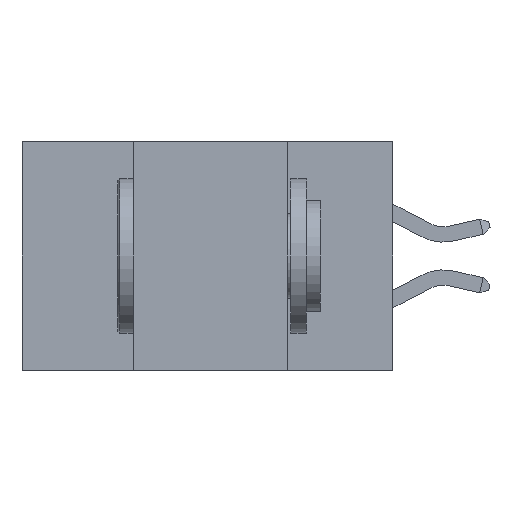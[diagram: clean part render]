
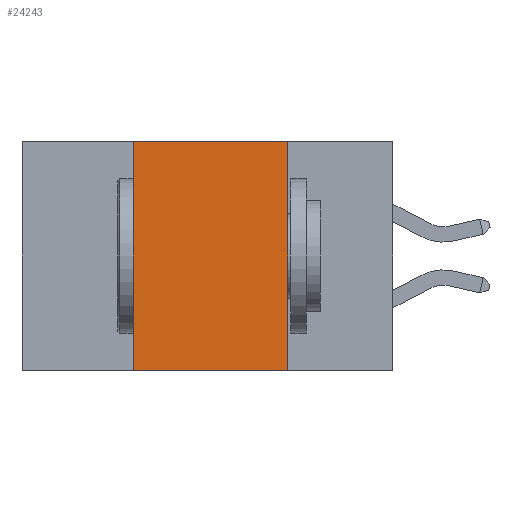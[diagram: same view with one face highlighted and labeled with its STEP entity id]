
A CAD part, left-side view. The second image highlights one B-rep face of the part: STEP entity #24243.
In plain terms, the highlighted planar face has unit normal (-1, 0, 0).
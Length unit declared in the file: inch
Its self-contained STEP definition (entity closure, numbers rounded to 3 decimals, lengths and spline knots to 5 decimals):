
#56 = CARTESIAN_POINT ( 'NONE',  ( 0., 0.42, 0. ) ) ;
#377 = CARTESIAN_POINT ( 'NONE',  ( 0., 0.17, 0. ) ) ;
#559 = VERTEX_POINT ( 'NONE', #10148 ) ;
#649 = DIRECTION ( 'NONE',  ( 0., 0., -1. ) ) ;
#823 = EDGE_CURVE ( 'NONE', #21003, #13981, #11745, .T. ) ;
#1672 = EDGE_LOOP ( 'NONE', ( #23677, #8343, #2283, #2668 ) ) ;
#2136 = VECTOR ( 'NONE', #13683, 39.37008 ) ;
#2283 = ORIENTED_EDGE ( 'NONE', *, *, #8239, .F. ) ;
#2332 = EDGE_CURVE ( 'NONE', #13981, #14067, #5359, .T. ) ;
#2668 = ORIENTED_EDGE ( 'NONE', *, *, #18208, .T. ) ;
#5359 = LINE ( 'NONE', #12153, #21860 ) ;
#5470 = LINE ( 'NONE', #9801, #2136 ) ;
#6716 = CARTESIAN_POINT ( 'NONE',  ( 0., 0.6, 0. ) ) ;
#8239 = EDGE_CURVE ( 'NONE', #559, #21003, #8372, .T. ) ;
#8265 = CARTESIAN_POINT ( 'NONE',  ( 0., 0.42, 0. ) ) ;
#8291 = DIRECTION ( 'NONE',  ( 0., 0., 1. ) ) ;
#8343 = ORIENTED_EDGE ( 'NONE', *, *, #823, .F. ) ;
#8372 = LINE ( 'NONE', #56, #14719 ) ;
#9257 = FACE_OUTER_BOUND ( 'NONE', #1672, .T. ) ;
#9801 = CARTESIAN_POINT ( 'NONE',  ( 0., 0.6, -0.37 ) ) ;
#10148 = CARTESIAN_POINT ( 'NONE',  ( 0., 0.42, -0.37 ) ) ;
#11745 = LINE ( 'NONE', #6716, #16259 ) ;
#12153 = CARTESIAN_POINT ( 'NONE',  ( 0., 0.17, 0. ) ) ;
#13683 = DIRECTION ( 'NONE',  ( 0., -1., 0. ) ) ;
#13981 = VERTEX_POINT ( 'NONE', #377 ) ;
#14067 = VERTEX_POINT ( 'NONE', #16269 ) ;
#14719 = VECTOR ( 'NONE', #8291, 39.37008 ) ;
#16259 = VECTOR ( 'NONE', #20141, 39.37008 ) ;
#16269 = CARTESIAN_POINT ( 'NONE',  ( 0., 0.17, -0.37 ) ) ;
#18208 = EDGE_CURVE ( 'NONE', #559, #14067, #5470, .T. ) ;
#18315 = DIRECTION ( 'NONE',  ( 1., 0., 0. ) ) ;
#20141 = DIRECTION ( 'NONE',  ( 0., -1., 0. ) ) ;
#21003 = VERTEX_POINT ( 'NONE', #8265 ) ;
#21140 = AXIS2_PLACEMENT_3D ( 'NONE', #23816, #18315, #24077 ) ;
#21860 = VECTOR ( 'NONE', #649, 39.37008 ) ;
#23677 = ORIENTED_EDGE ( 'NONE', *, *, #2332, .F. ) ;
#23816 = CARTESIAN_POINT ( 'NONE',  ( 0., 0.6, 0. ) ) ;
#23983 = PLANE ( 'NONE',  #21140 ) ;
#24077 = DIRECTION ( 'NONE',  ( 0., 0., -1. ) ) ;
#24243 = ADVANCED_FACE ( 'NONE', ( #9257 ), #23983, .F. ) ;
